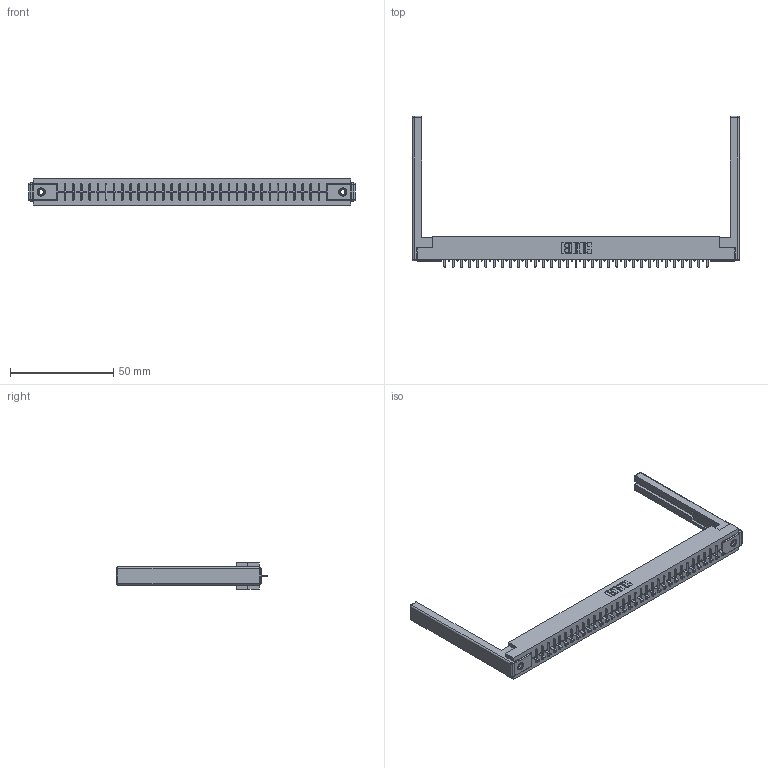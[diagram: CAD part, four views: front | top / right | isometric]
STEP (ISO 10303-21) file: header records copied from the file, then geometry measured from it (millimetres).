
FILE_DESCRIPTION (( 'STEP AP203' ), '1' );
FILE_NAME ('306-033-421-168.STEP', '2020-09-22T03:02:52', ( '' ), ( '' ), 'SwSTEP 2.0', 'SolidWorks 2020', '' );
FILE_SCHEMA (( 'CONFIG_CONTROL_DESIGN' ));
Length unit declared in the file: inch
Products named in the file (5): 345-250-001_345-250-001-102; 306 Part_.156 Dia; 307-220-068; 306-033-421-168; 306-290-001_121
Assembly tree (38 placements, depth 2):
  306-033-421-168
    306 Part_.156 Dia
    306-290-001_121  x33
    345-250-001_345-250-001-102  x2
    307-220-068  x2
Bounding box: 158.19 x 73.18 x 12.7 mm (x, y, z)
Volume: 21729.3 mm3; surface area: 21551.6 mm2
Topology: 38 solids, 38 shells, 2580 faces, 7207 edges, 4606 vertices
Faces by surface type: plane 1707, cylinder 717, sphere 140, cone 12, torus 4
Entity records: 34655 total; most frequent: CARTESIAN_POINT 5783, ORIENTED_EDGE 5724, DIRECTION 5716, EDGE_CURVE 2862, LINE 2230, VECTOR 2230, VERTEX_POINT 1810, AXIS2_PLACEMENT_3D 1743
